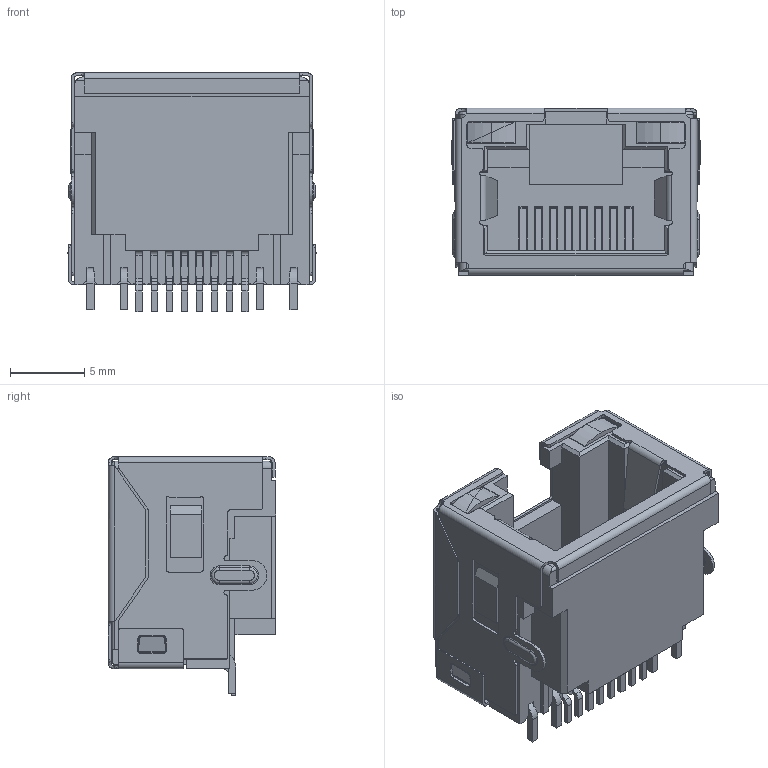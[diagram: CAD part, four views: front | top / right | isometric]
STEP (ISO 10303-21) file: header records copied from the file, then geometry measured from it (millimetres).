
FILE_DESCRIPTION (( 'STEP AP203' ), '1' );
FILE_NAME ('J6E018824L51110.STEP', '2020-03-19T14:25:04', ( '' ), ( '' ), 'SwSTEP 2.0', 'SolidWorks 2016', '' );
FILE_SCHEMA (( 'CONFIG_CONTROL_DESIGN' ));
Length unit declared in the file: millimetre
Products named in the file (6): 6E Insulator_LED; 6E LED LH_5-Green-Yellow; 6E Shield_LED; 6E Contacts; 6E LED RH_1-Yellow; J6E018824L51110
Assembly tree (5 placements, depth 2):
  J6E018824L51110
    6E Insulator_LED
    6E Contacts
    6E Shield_LED
    6E LED LH_5-Green-Yellow
    6E LED RH_1-Yellow
Bounding box: 16.75 x 11.3 x 16.15 mm (x, y, z)
Volume: 1109.4 mm3; surface area: 4045.2 mm2
Topology: 12 solids, 12 shells, 1498 faces, 4208 edges, 2727 vertices
Faces by surface type: plane 1099, cylinder 349, bspline 50
Entity records: 50396 total; most frequent: CARTESIAN_POINT 11133, ORIENTED_EDGE 8416, DIRECTION 7567, EDGE_CURVE 4208, VECTOR 3385, LINE 3385, VERTEX_POINT 2727, AXIS2_PLACEMENT_3D 2091
